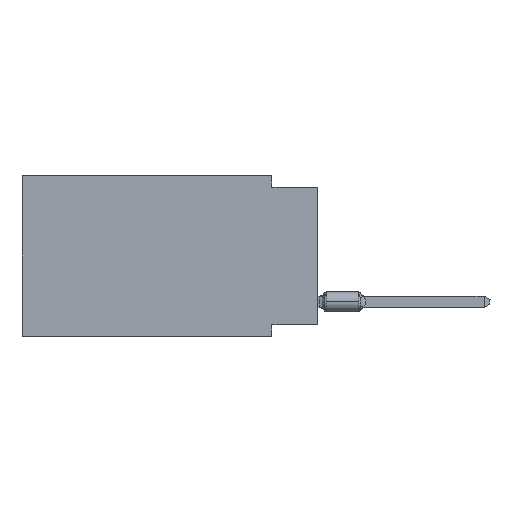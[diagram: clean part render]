
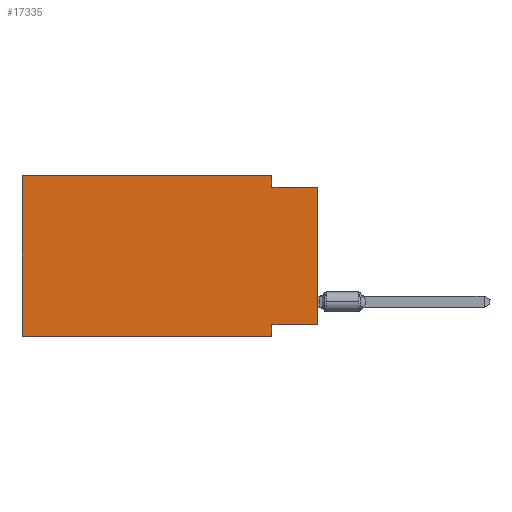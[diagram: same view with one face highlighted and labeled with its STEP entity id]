
A CAD part, left-side view. The second image highlights one B-rep face of the part: STEP entity #17335.
In plain terms, the highlighted planar face has unit normal (-1, 0, 0).
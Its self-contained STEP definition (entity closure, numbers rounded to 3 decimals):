
#3031 = ORIENTED_EDGE ( 'NONE', *, *, #7698, .T. ) ;
#3091 = EDGE_CURVE ( 'NONE', #19264, #41642, #36786, .T. ) ;
#4358 = CARTESIAN_POINT ( 'NONE',  ( 0., 16.383, 0. ) ) ;
#5555 = VECTOR ( 'NONE', #6445, 1000. ) ;
#6113 = CARTESIAN_POINT ( 'NONE',  ( 0., 2.54, 0. ) ) ;
#6179 = CARTESIAN_POINT ( 'NONE',  ( 0., 16.383, -8.89 ) ) ;
#6445 = DIRECTION ( 'NONE',  ( 0., -1., 0. ) ) ;
#6535 = CARTESIAN_POINT ( 'NONE',  ( 0., 0., -8.255 ) ) ;
#7039 = CARTESIAN_POINT ( 'NONE',  ( 0., 2.54, -8.89 ) ) ;
#7698 = EDGE_CURVE ( 'NONE', #41442, #36506, #12863, .T. ) ;
#8705 = VECTOR ( 'NONE', #38964, 1000. ) ;
#10401 = VERTEX_POINT ( 'NONE', #37929 ) ;
#10886 = ORIENTED_EDGE ( 'NONE', *, *, #42261, .T. ) ;
#11038 = CARTESIAN_POINT ( 'NONE',  ( 0., 0., -8.255 ) ) ;
#11322 = EDGE_LOOP ( 'NONE', ( #10886, #34293, #33916, #12160, #39059, #3031, #12992, #19057 ) ) ;
#12034 = EDGE_CURVE ( 'NONE', #41442, #26478, #23759, .T. ) ;
#12160 = ORIENTED_EDGE ( 'NONE', *, *, #24984, .F. ) ;
#12566 = PLANE ( 'NONE',  #18317 ) ;
#12863 = LINE ( 'NONE', #40204, #5555 ) ;
#12992 = ORIENTED_EDGE ( 'NONE', *, *, #15075, .F. ) ;
#14060 = LINE ( 'NONE', #19798, #16450 ) ;
#15075 = EDGE_CURVE ( 'NONE', #41642, #36506, #29490, .T. ) ;
#16450 = VECTOR ( 'NONE', #20015, 1000. ) ;
#17335 = ADVANCED_FACE ( 'NONE', ( #19403 ), #12566, .F. ) ;
#17640 = CARTESIAN_POINT ( 'NONE',  ( 0., 2.54, -8.255 ) ) ;
#18317 = AXIS2_PLACEMENT_3D ( 'NONE', #29334, #35970, #42786 ) ;
#19057 = ORIENTED_EDGE ( 'NONE', *, *, #3091, .F. ) ;
#19264 = VERTEX_POINT ( 'NONE', #11038 ) ;
#19338 = VECTOR ( 'NONE', #37002, 1000. ) ;
#19403 = FACE_OUTER_BOUND ( 'NONE', #11322, .T. ) ;
#19532 = LINE ( 'NONE', #38743, #8705 ) ;
#19781 = LINE ( 'NONE', #6113, #29108 ) ;
#19798 = CARTESIAN_POINT ( 'NONE',  ( 0., 0., 0. ) ) ;
#20003 = DIRECTION ( 'NONE',  ( 0., 0., -1. ) ) ;
#20015 = DIRECTION ( 'NONE',  ( 0., 0., 1. ) ) ;
#20671 = CARTESIAN_POINT ( 'NONE',  ( 0., 16.383, 0. ) ) ;
#23169 = VECTOR ( 'NONE', #24855, 1000. ) ;
#23415 = VERTEX_POINT ( 'NONE', #37739 ) ;
#23759 = LINE ( 'NONE', #20671, #33133 ) ;
#24432 = LINE ( 'NONE', #4358, #23169 ) ;
#24855 = DIRECTION ( 'NONE',  ( 0., -1., 0. ) ) ;
#24984 = EDGE_CURVE ( 'NONE', #26478, #26861, #24432, .T. ) ;
#25753 = DIRECTION ( 'NONE',  ( 0., 0., -1. ) ) ;
#26478 = VERTEX_POINT ( 'NONE', #35233 ) ;
#26861 = VERTEX_POINT ( 'NONE', #41945 ) ;
#29108 = VECTOR ( 'NONE', #20003, 1000. ) ;
#29334 = CARTESIAN_POINT ( 'NONE',  ( 0., 16.383, 0. ) ) ;
#29490 = LINE ( 'NONE', #35695, #34444 ) ;
#30611 = DIRECTION ( 'NONE',  ( 0., 0., 1. ) ) ;
#33133 = VECTOR ( 'NONE', #30611, 1000. ) ;
#33916 = ORIENTED_EDGE ( 'NONE', *, *, #35174, .F. ) ;
#34293 = ORIENTED_EDGE ( 'NONE', *, *, #42474, .F. ) ;
#34444 = VECTOR ( 'NONE', #25753, 1000. ) ;
#35174 = EDGE_CURVE ( 'NONE', #26861, #10401, #19781, .T. ) ;
#35233 = CARTESIAN_POINT ( 'NONE',  ( 0., 16.383, 0. ) ) ;
#35695 = CARTESIAN_POINT ( 'NONE',  ( 0., 2.54, -8.89 ) ) ;
#35970 = DIRECTION ( 'NONE',  ( 1., 0., 0. ) ) ;
#36506 = VERTEX_POINT ( 'NONE', #7039 ) ;
#36786 = LINE ( 'NONE', #6535, #19338 ) ;
#37002 = DIRECTION ( 'NONE',  ( 0., 1., 0. ) ) ;
#37739 = CARTESIAN_POINT ( 'NONE',  ( 0., 0., -0.635 ) ) ;
#37929 = CARTESIAN_POINT ( 'NONE',  ( 0., 2.54, -0.635 ) ) ;
#38743 = CARTESIAN_POINT ( 'NONE',  ( 0., 0., -0.635 ) ) ;
#38964 = DIRECTION ( 'NONE',  ( 0., -1., 0. ) ) ;
#39059 = ORIENTED_EDGE ( 'NONE', *, *, #12034, .F. ) ;
#40204 = CARTESIAN_POINT ( 'NONE',  ( 0., 16.383, -8.89 ) ) ;
#41442 = VERTEX_POINT ( 'NONE', #6179 ) ;
#41642 = VERTEX_POINT ( 'NONE', #17640 ) ;
#41945 = CARTESIAN_POINT ( 'NONE',  ( 0., 2.54, 0. ) ) ;
#42261 = EDGE_CURVE ( 'NONE', #19264, #23415, #14060, .T. ) ;
#42474 = EDGE_CURVE ( 'NONE', #10401, #23415, #19532, .T. ) ;
#42786 = DIRECTION ( 'NONE',  ( 0., 0., -1. ) ) ;
